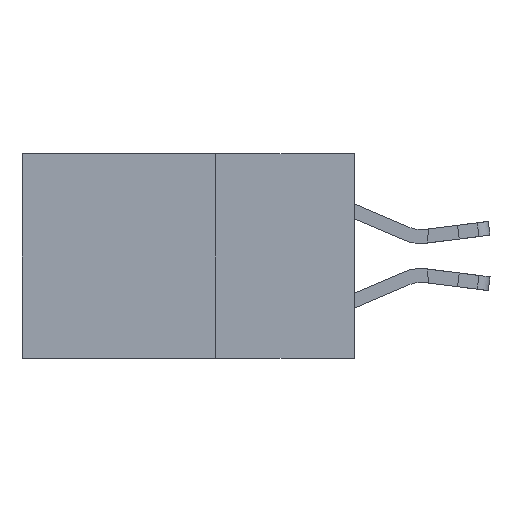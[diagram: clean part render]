
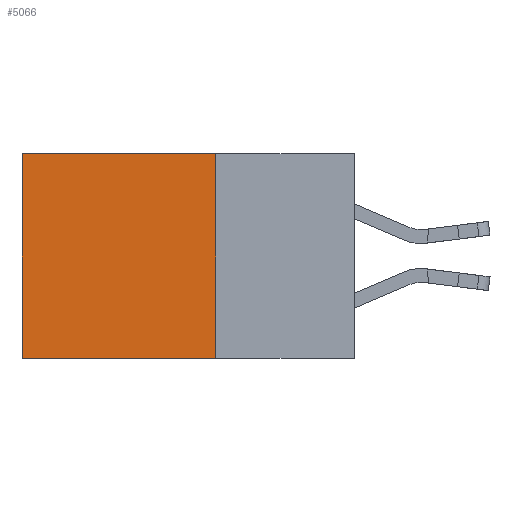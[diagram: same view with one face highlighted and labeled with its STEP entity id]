
A CAD part, left-side view. The second image highlights one B-rep face of the part: STEP entity #5066.
In plain terms, the highlighted planar face has unit normal (-1, 0, 0).
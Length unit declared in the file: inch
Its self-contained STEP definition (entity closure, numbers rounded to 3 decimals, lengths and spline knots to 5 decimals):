
#172 = DIRECTION ( 'NONE',  ( 0., 1., 0. ) ) ;
#226 = CARTESIAN_POINT ( 'NONE',  ( 0.2615, 0.25, -0.37 ) ) ;
#392 = CARTESIAN_POINT ( 'NONE',  ( 0.2615, 0.6, -0.37 ) ) ;
#828 = EDGE_CURVE ( 'NONE', #10738, #15426, #8571, .T. ) ;
#1434 = VERTEX_POINT ( 'NONE', #1774 ) ;
#1513 = ORIENTED_EDGE ( 'NONE', *, *, #9888, .F. ) ;
#1774 = CARTESIAN_POINT ( 'NONE',  ( 0.2615, 0.25, 0. ) ) ;
#2316 = EDGE_CURVE ( 'NONE', #1434, #10738, #5329, .T. ) ;
#2864 = EDGE_CURVE ( 'NONE', #1434, #12802, #3824, .T. ) ;
#2942 = AXIS2_PLACEMENT_3D ( 'NONE', #10276, #11427, #11439 ) ;
#3824 = LINE ( 'NONE', #12537, #13389 ) ;
#4468 = CARTESIAN_POINT ( 'NONE',  ( 0.2615, 0.25, 0. ) ) ;
#4640 = EDGE_LOOP ( 'NONE', ( #9726, #1513, #14475, #15062 ) ) ;
#4851 = DIRECTION ( 'NONE',  ( 0., 1., 0. ) ) ;
#5066 = ADVANCED_FACE ( 'NONE', ( #10537 ), #11626, .F. ) ;
#5329 = LINE ( 'NONE', #4468, #11368 ) ;
#5369 = VECTOR ( 'NONE', #8079, 39.37008 ) ;
#8079 = DIRECTION ( 'NONE',  ( 0., 0., -1. ) ) ;
#8347 = DIRECTION ( 'NONE',  ( 0., 0., -1. ) ) ;
#8571 = LINE ( 'NONE', #392, #5369 ) ;
#9150 = CARTESIAN_POINT ( 'NONE',  ( 0.2615, 0.6, -0.37 ) ) ;
#9726 = ORIENTED_EDGE ( 'NONE', *, *, #828, .T. ) ;
#9727 = CARTESIAN_POINT ( 'NONE',  ( 0.2615, 0.6, 0. ) ) ;
#9888 = EDGE_CURVE ( 'NONE', #12802, #15426, #11102, .T. ) ;
#9961 = VECTOR ( 'NONE', #172, 39.37008 ) ;
#10276 = CARTESIAN_POINT ( 'NONE',  ( 0.2615, 0.25, -0.37 ) ) ;
#10537 = FACE_OUTER_BOUND ( 'NONE', #4640, .T. ) ;
#10738 = VERTEX_POINT ( 'NONE', #9727 ) ;
#11102 = LINE ( 'NONE', #226, #9961 ) ;
#11105 = CARTESIAN_POINT ( 'NONE',  ( 0.2615, 0.25, -0.37 ) ) ;
#11368 = VECTOR ( 'NONE', #4851, 39.37008 ) ;
#11427 = DIRECTION ( 'NONE',  ( 1., 0., 0. ) ) ;
#11439 = DIRECTION ( 'NONE',  ( 0., 0., -1. ) ) ;
#11626 = PLANE ( 'NONE',  #2942 ) ;
#12537 = CARTESIAN_POINT ( 'NONE',  ( 0.2615, 0.25, -0.37 ) ) ;
#12802 = VERTEX_POINT ( 'NONE', #11105 ) ;
#13389 = VECTOR ( 'NONE', #8347, 39.37008 ) ;
#14475 = ORIENTED_EDGE ( 'NONE', *, *, #2864, .F. ) ;
#15062 = ORIENTED_EDGE ( 'NONE', *, *, #2316, .T. ) ;
#15426 = VERTEX_POINT ( 'NONE', #9150 ) ;
